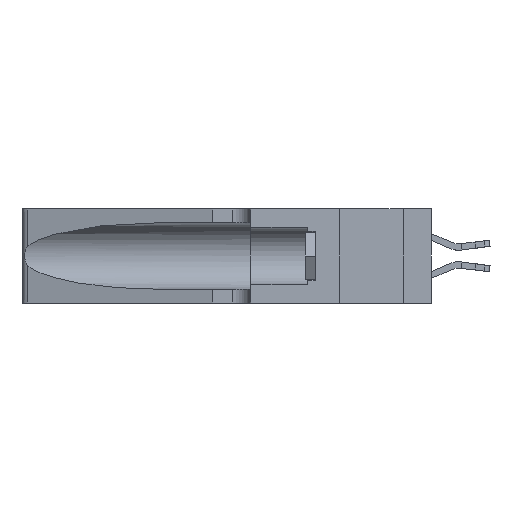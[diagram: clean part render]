
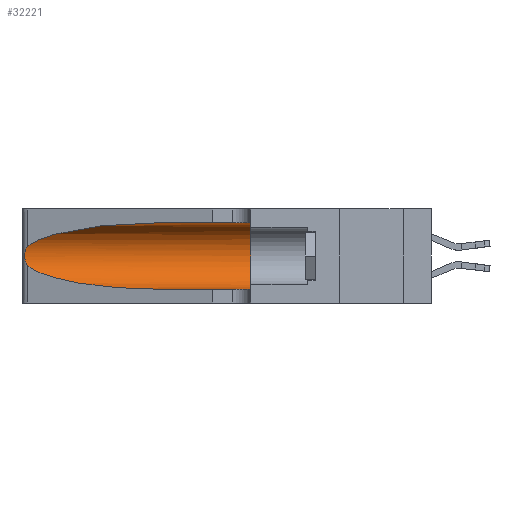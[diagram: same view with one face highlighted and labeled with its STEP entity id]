
A CAD part, left-side view. The second image highlights one B-rep face of the part: STEP entity #32221.
In plain terms, the highlighted cylindrical face has radius 3.308 mm (diameter 6.617 mm), a partial arc.
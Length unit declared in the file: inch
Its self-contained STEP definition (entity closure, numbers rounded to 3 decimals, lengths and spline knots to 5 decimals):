
#966 = CARTESIAN_POINT ( 'NONE',  ( 0.25487, 1.22718, 0.22369 ) ) ;
#1084 = CARTESIAN_POINT ( 'NONE',  ( 0.25487, 1.22718, 0.14631 ) ) ;
#1298 = CYLINDRICAL_SURFACE ( 'NONE', #11252, 0.13025 ) ;
#1464 = CARTESIAN_POINT ( 'NONE',  ( 0.1305, 0.35, 0.31525 ) ) ;
#1555 = VERTEX_POINT ( 'NONE', #25949 ) ;
#1829 = EDGE_CURVE ( 'NONE', #22492, #1555, #18385, .T. ) ;
#1930 = VERTEX_POINT ( 'NONE', #16853 ) ;
#2690 = EDGE_LOOP ( 'NONE', ( #13225, #20258, #7014, #30487, #10320, #11974 ) ) ;
#3722 = CARTESIAN_POINT ( 'NONE',  ( 0.25639, 1.23184, 0.21858 ) ) ;
#5548 = DIRECTION ( 'NONE',  ( 0., 1., 0. ) ) ;
#6356 = DIRECTION ( 'NONE',  ( 0., 0., -1. ) ) ;
#6416 = CARTESIAN_POINT ( 'NONE',  ( 0.25854, 1.2359, 0.20912 ) ) ;
#6669 = DIRECTION ( 'NONE',  ( 0., -1., 0. ) ) ;
#7014 = ORIENTED_EDGE ( 'NONE', *, *, #1829, .T. ) ;
#7896 = CARTESIAN_POINT ( 'NONE',  ( 0.1305, 0.35, 0.05475 ) ) ;
#8280 = AXIS2_PLACEMENT_3D ( 'NONE', #21378, #5548, #24013 ) ;
#8517 = CARTESIAN_POINT ( 'NONE',  ( 0.18966, 0.96281, 0.05475 ) ) ;
#8585 = LINE ( 'NONE', #27748, #14822 ) ;
#9070 = CARTESIAN_POINT ( 'NONE',  ( 0.26075, 1.23896, 0.19203 ) ) ;
#9688 = VERTEX_POINT ( 'NONE', #1464 ) ;
#9984 = VERTEX_POINT ( 'NONE', #7896 ) ;
#10108 = VECTOR ( 'NONE', #20772, 39.37008 ) ;
#10320 = ORIENTED_EDGE ( 'NONE', *, *, #15712, .F. ) ;
#10325 = CARTESIAN_POINT ( 'NONE',  ( 0.25487, 1.22718, 0.22369 ) ) ;
#11252 = AXIS2_PLACEMENT_3D ( 'NONE', #16878, #22167, #6356 ) ;
#11746 = CARTESIAN_POINT ( 'NONE',  ( 0.26017, 1.23833, 0.17102 ) ) ;
#11974 = ORIENTED_EDGE ( 'NONE', *, *, #13858, .F. ) ;
#12220 = CARTESIAN_POINT ( 'NONE',  ( 0.1305, 1.61858, 0.05475 ) ) ;
#13225 = ORIENTED_EDGE ( 'NONE', *, *, #31915, .T. ) ;
#13858 = EDGE_CURVE ( 'NONE', #31771, #9688, #8585, .T. ) ;
#14407 = CARTESIAN_POINT ( 'NONE',  ( 0.25789, 1.23486, 0.15765 ) ) ;
#14689 = CIRCLE ( 'NONE', #8280, 0.13025 ) ;
#14822 = VECTOR ( 'NONE', #6669, 39.37008 ) ;
#15499 = FACE_OUTER_BOUND ( 'NONE', #2690, .T. ) ;
#15712 = EDGE_CURVE ( 'NONE', #9688, #9984, #14689, .T. ) ;
#16391 = CARTESIAN_POINT ( 'NONE',  ( 0.2373, 1.15595, 0.08982 ) ) ;
#16751 = EDGE_CURVE ( 'NONE', #1555, #9984, #24118, .T. ) ;
#16853 = CARTESIAN_POINT ( 'NONE',  ( 0.25487, 1.22718, 0.22369 ) ) ;
#16878 = CARTESIAN_POINT ( 'NONE',  ( 0.1305, 1.61858, 0.185 ) ) ;
#17053 = CARTESIAN_POINT ( 'NONE',  ( 0.25555, 1.22993, 0.14849 ) ) ;
#18385 =( BOUNDED_CURVE ( )  B_SPLINE_CURVE ( 3, ( #19057, #16391, #8517, #26955 ),
 .UNSPECIFIED., .F., .T. ) 
 B_SPLINE_CURVE_WITH_KNOTS ( ( 4, 4 ),
 ( 3.44316, 4.71239 ),
 .UNSPECIFIED. ) 
 CURVE ( )  GEOMETRIC_REPRESENTATION_ITEM ( )  RATIONAL_B_SPLINE_CURVE ( ( 1., 0.87, 0.87, 1. ) ) 
 REPRESENTATION_ITEM ( '' )  );
#18524 =( BOUNDED_CURVE ( )  B_SPLINE_CURVE ( 3, ( #20839, #33868, #26096, #10325 ),
 .UNSPECIFIED., .F., .T. ) 
 B_SPLINE_CURVE_WITH_KNOTS ( ( 4, 4 ),
 ( 1.5708, 2.84003 ),
 .UNSPECIFIED. ) 
 CURVE ( )  GEOMETRIC_REPRESENTATION_ITEM ( )  RATIONAL_B_SPLINE_CURVE ( ( 1., 0.87, 0.87, 1. ) ) 
 REPRESENTATION_ITEM ( '' )  );
#19057 = CARTESIAN_POINT ( 'NONE',  ( 0.25487, 1.22718, 0.14631 ) ) ;
#20258 = ORIENTED_EDGE ( 'NONE', *, *, #25554, .T. ) ;
#20772 = DIRECTION ( 'NONE',  ( 0., -1., 0. ) ) ;
#20839 = CARTESIAN_POINT ( 'NONE',  ( 0.1305, 0.72297, 0.31525 ) ) ;
#21378 = CARTESIAN_POINT ( 'NONE',  ( 0.1305, 0.35, 0.185 ) ) ;
#22167 = DIRECTION ( 'NONE',  ( 0., -1., 0. ) ) ;
#22226 = CARTESIAN_POINT ( 'NONE',  ( 0.25787, 1.23484, 0.2124 ) ) ;
#22492 = VERTEX_POINT ( 'NONE', #27282 ) ;
#24013 = DIRECTION ( 'NONE',  ( 0., 0., 1. ) ) ;
#24118 = LINE ( 'NONE', #12220, #10108 ) ;
#24759 = CARTESIAN_POINT ( 'NONE',  ( 0.25555, 1.22994, 0.2215 ) ) ;
#24867 = CARTESIAN_POINT ( 'NONE',  ( 0.26018, 1.23835, 0.19895 ) ) ;
#25554 = EDGE_CURVE ( 'NONE', #1930, #22492, #26568, .T. ) ;
#25949 = CARTESIAN_POINT ( 'NONE',  ( 0.1305, 0.72297, 0.05475 ) ) ;
#26096 = CARTESIAN_POINT ( 'NONE',  ( 0.2373, 1.15595, 0.28018 ) ) ;
#26568 = B_SPLINE_CURVE_WITH_KNOTS ( 'NONE', 3,
 ( #966, #24759, #3722, #22226, #6416, #24867, #9070, #27494, #11746, #30134, #14407, #32753, #17053, #1084 ),
 .UNSPECIFIED., .F., .F.,
 ( 4, 2, 2, 2, 2, 2, 4 ),
 ( 0., 0.00027, 0.00053, 0.00107, 0.0016, 0.00187, 0.00214 ),
 .UNSPECIFIED. ) ;
#26955 = CARTESIAN_POINT ( 'NONE',  ( 0.1305, 0.72297, 0.05475 ) ) ;
#27282 = CARTESIAN_POINT ( 'NONE',  ( 0.25487, 1.22718, 0.14631 ) ) ;
#27494 = CARTESIAN_POINT ( 'NONE',  ( 0.26075, 1.23896, 0.178 ) ) ;
#27748 = CARTESIAN_POINT ( 'NONE',  ( 0.1305, 1.61858, 0.31525 ) ) ;
#30134 = CARTESIAN_POINT ( 'NONE',  ( 0.25856, 1.23593, 0.16098 ) ) ;
#30487 = ORIENTED_EDGE ( 'NONE', *, *, #16751, .T. ) ;
#30687 = CARTESIAN_POINT ( 'NONE',  ( 0.1305, 0.72297, 0.31525 ) ) ;
#31771 = VERTEX_POINT ( 'NONE', #30687 ) ;
#31915 = EDGE_CURVE ( 'NONE', #31771, #1930, #18524, .T. ) ;
#32221 = ADVANCED_FACE ( 'NONE', ( #15499 ), #1298, .F. ) ;
#32753 = CARTESIAN_POINT ( 'NONE',  ( 0.25639, 1.23186, 0.15144 ) ) ;
#33868 = CARTESIAN_POINT ( 'NONE',  ( 0.18966, 0.96281, 0.31525 ) ) ;
